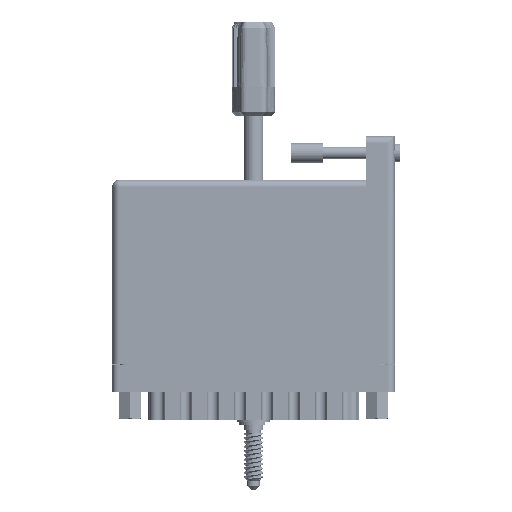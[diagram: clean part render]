
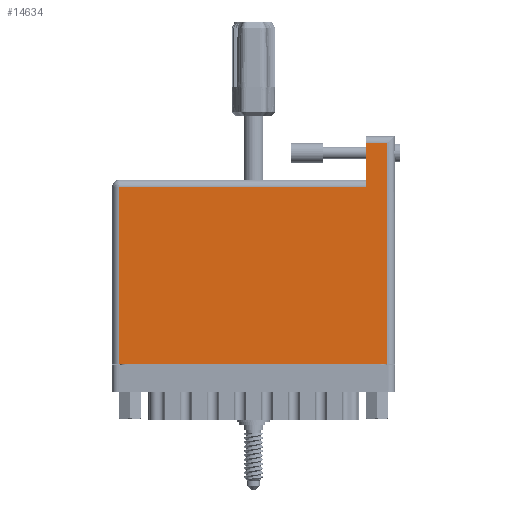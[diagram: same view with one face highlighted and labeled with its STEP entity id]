
A CAD part, front view. The second image highlights one B-rep face of the part: STEP entity #14634.
In plain terms, the highlighted face is planar.
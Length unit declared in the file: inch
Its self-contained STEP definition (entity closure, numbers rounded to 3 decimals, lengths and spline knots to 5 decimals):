
#118 = LINE ( 'NONE', #53563, #32367 ) ;
#162 = ORIENTED_EDGE ( 'NONE', *, *, #42230, .T. ) ;
#2322 = LINE ( 'NONE', #66541, #50083 ) ;
#2807 = DIRECTION ( 'NONE',  ( 1., 0., 0. ) ) ;
#3563 = DIRECTION ( 'NONE',  ( 0., -1., 0. ) ) ;
#3944 = VECTOR ( 'NONE', #62492, 39.37008 ) ;
#5811 = DIRECTION ( 'NONE',  ( -1., 0., 0. ) ) ;
#10712 = CARTESIAN_POINT ( 'NONE',  ( 2.438, 2.125, 0. ) ) ;
#12601 = CARTESIAN_POINT ( 'NONE',  ( 0.07, 1.705, 0. ) ) ;
#14634 = ADVANCED_FACE ( 'NONE', ( #51356 ), #76037, .F. ) ;
#16370 = DIRECTION ( 'NONE',  ( -1., 0., 0. ) ) ;
#17121 = CARTESIAN_POINT ( 'NONE',  ( 2.648, 2.195, 0. ) ) ;
#22131 = EDGE_CURVE ( 'NONE', #71669, #29707, #84942, .T. ) ;
#23686 = DIRECTION ( 'NONE',  ( 0., 0., -1. ) ) ;
#23876 = VECTOR ( 'NONE', #38847, 39.37008 ) ;
#26772 = VECTOR ( 'NONE', #3563, 39.37008 ) ;
#28941 = VECTOR ( 'NONE', #56659, 39.37008 ) ;
#29707 = VERTEX_POINT ( 'NONE', #10712 ) ;
#31014 = CARTESIAN_POINT ( 'NONE',  ( 0., 1.775, 0. ) ) ;
#31152 = EDGE_CURVE ( 'NONE', #74375, #37498, #2322, .T. ) ;
#32367 = VECTOR ( 'NONE', #2807, 39.37008 ) ;
#35604 = EDGE_CURVE ( 'NONE', #37498, #78669, #47028, .T. ) ;
#37498 = VERTEX_POINT ( 'NONE', #12601 ) ;
#37597 = ORIENTED_EDGE ( 'NONE', *, *, #44905, .T. ) ;
#38847 = DIRECTION ( 'NONE',  ( 0., -1., 0. ) ) ;
#42230 = EDGE_CURVE ( 'NONE', #54492, #71669, #85060, .T. ) ;
#44328 = ORIENTED_EDGE ( 'NONE', *, *, #31152, .T. ) ;
#44905 = EDGE_CURVE ( 'NONE', #29707, #74375, #70502, .T. ) ;
#47028 = LINE ( 'NONE', #94883, #26772 ) ;
#48484 = CARTESIAN_POINT ( 'NONE',  ( 2.648, 2.125, 0. ) ) ;
#50083 = VECTOR ( 'NONE', #5811, 39.37008 ) ;
#51356 = FACE_OUTER_BOUND ( 'NONE', #57536, .T. ) ;
#53563 = CARTESIAN_POINT ( 'NONE',  ( 0., 0., 0. ) ) ;
#54492 = VERTEX_POINT ( 'NONE', #58866 ) ;
#56659 = DIRECTION ( 'NONE',  ( -1., 0., 0. ) ) ;
#57536 = EDGE_LOOP ( 'NONE', ( #44328, #71088, #61532, #162, #71939, #37597 ) ) ;
#58866 = CARTESIAN_POINT ( 'NONE',  ( 2.648, 0., 0. ) ) ;
#61532 = ORIENTED_EDGE ( 'NONE', *, *, #79352, .T. ) ;
#62492 = DIRECTION ( 'NONE',  ( 0., 1., 0. ) ) ;
#63347 = CARTESIAN_POINT ( 'NONE',  ( 0., 2.125, 0. ) ) ;
#66541 = CARTESIAN_POINT ( 'NONE',  ( 0., 1.705, 0. ) ) ;
#69640 = CARTESIAN_POINT ( 'NONE',  ( 0.07, 0., 0. ) ) ;
#70502 = LINE ( 'NONE', #77166, #23876 ) ;
#71088 = ORIENTED_EDGE ( 'NONE', *, *, #35604, .T. ) ;
#71669 = VERTEX_POINT ( 'NONE', #48484 ) ;
#71939 = ORIENTED_EDGE ( 'NONE', *, *, #22131, .T. ) ;
#74375 = VERTEX_POINT ( 'NONE', #93710 ) ;
#76037 = PLANE ( 'NONE',  #94127 ) ;
#77166 = CARTESIAN_POINT ( 'NONE',  ( 2.438, 2.195, 0. ) ) ;
#78669 = VERTEX_POINT ( 'NONE', #69640 ) ;
#79352 = EDGE_CURVE ( 'NONE', #78669, #54492, #118, .T. ) ;
#84942 = LINE ( 'NONE', #63347, #28941 ) ;
#85060 = LINE ( 'NONE', #17121, #3944 ) ;
#93710 = CARTESIAN_POINT ( 'NONE',  ( 2.438, 1.705, 0. ) ) ;
#94127 = AXIS2_PLACEMENT_3D ( 'NONE', #31014, #23686, #16370 ) ;
#94883 = CARTESIAN_POINT ( 'NONE',  ( 0.07, 0., 0. ) ) ;
